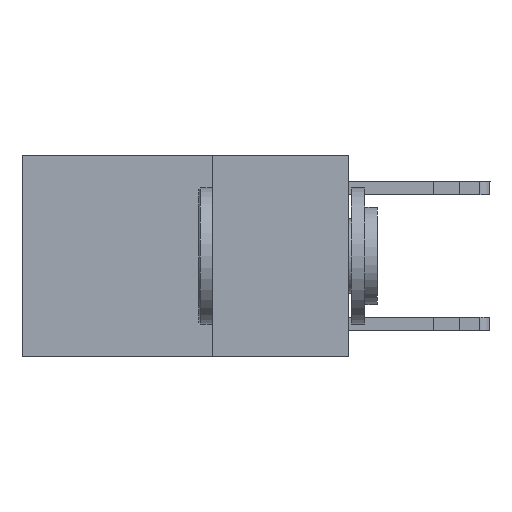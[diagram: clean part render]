
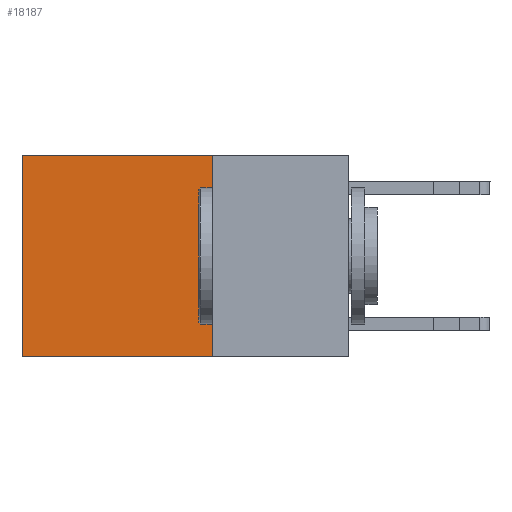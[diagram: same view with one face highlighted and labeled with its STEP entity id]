
A CAD part, left-side view. The second image highlights one B-rep face of the part: STEP entity #18187.
In plain terms, the highlighted planar face has unit normal (-1, 0, 0).
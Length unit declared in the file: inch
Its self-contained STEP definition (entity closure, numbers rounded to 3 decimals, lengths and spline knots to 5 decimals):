
#647 = VECTOR ( 'NONE', #19453, 39.37008 ) ;
#782 = VECTOR ( 'NONE', #16956, 39.37008 ) ;
#1092 = LINE ( 'NONE', #6745, #647 ) ;
#2630 = VECTOR ( 'NONE', #12367, 39.37008 ) ;
#2915 = CARTESIAN_POINT ( 'NONE',  ( 0.2625, 0.25, 0. ) ) ;
#3266 = VERTEX_POINT ( 'NONE', #7715 ) ;
#3829 = CARTESIAN_POINT ( 'NONE',  ( 0.2625, 0.6, 0. ) ) ;
#4664 = ORIENTED_EDGE ( 'NONE', *, *, #22046, .T. ) ;
#6486 = CARTESIAN_POINT ( 'NONE',  ( 0.2625, 0.25, -0.37 ) ) ;
#6581 = EDGE_CURVE ( 'NONE', #9595, #10878, #1092, .T. ) ;
#6668 = ORIENTED_EDGE ( 'NONE', *, *, #14775, .F. ) ;
#6745 = CARTESIAN_POINT ( 'NONE',  ( 0.2625, 0.25, 0. ) ) ;
#7245 = DIRECTION ( 'NONE',  ( 0., 0., -1. ) ) ;
#7416 = CARTESIAN_POINT ( 'NONE',  ( 0.2625, 0.25, 0. ) ) ;
#7715 = CARTESIAN_POINT ( 'NONE',  ( 0.2625, 0.6, -0.37 ) ) ;
#9595 = VERTEX_POINT ( 'NONE', #7416 ) ;
#10083 = DIRECTION ( 'NONE',  ( 1., 0., 0. ) ) ;
#10477 = EDGE_CURVE ( 'NONE', #13343, #3266, #14534, .T. ) ;
#10878 = VERTEX_POINT ( 'NONE', #12613 ) ;
#11609 = EDGE_LOOP ( 'NONE', ( #12821, #6668, #11644, #4664 ) ) ;
#11644 = ORIENTED_EDGE ( 'NONE', *, *, #6581, .F. ) ;
#11858 = FACE_OUTER_BOUND ( 'NONE', #11609, .T. ) ;
#12367 = DIRECTION ( 'NONE',  ( 0., 1., 0. ) ) ;
#12613 = CARTESIAN_POINT ( 'NONE',  ( 0.2625, 0.25, -0.37 ) ) ;
#12821 = ORIENTED_EDGE ( 'NONE', *, *, #10477, .T. ) ;
#12929 = VECTOR ( 'NONE', #7245, 39.37008 ) ;
#13343 = VERTEX_POINT ( 'NONE', #18148 ) ;
#14534 = LINE ( 'NONE', #3829, #12929 ) ;
#14775 = EDGE_CURVE ( 'NONE', #10878, #3266, #17075, .T. ) ;
#15564 = LINE ( 'NONE', #17214, #2630 ) ;
#15858 = AXIS2_PLACEMENT_3D ( 'NONE', #2915, #10083, #20453 ) ;
#16913 = PLANE ( 'NONE',  #15858 ) ;
#16956 = DIRECTION ( 'NONE',  ( 0., 1., 0. ) ) ;
#17075 = LINE ( 'NONE', #6486, #782 ) ;
#17214 = CARTESIAN_POINT ( 'NONE',  ( 0.2625, 0.25, 0. ) ) ;
#18148 = CARTESIAN_POINT ( 'NONE',  ( 0.2625, 0.6, 0. ) ) ;
#18187 = ADVANCED_FACE ( 'NONE', ( #11858 ), #16913, .F. ) ;
#19453 = DIRECTION ( 'NONE',  ( 0., 0., -1. ) ) ;
#20453 = DIRECTION ( 'NONE',  ( 0., 0., -1. ) ) ;
#22046 = EDGE_CURVE ( 'NONE', #9595, #13343, #15564, .T. ) ;
